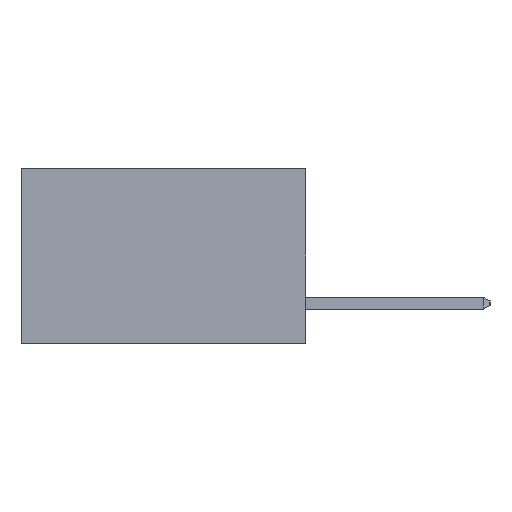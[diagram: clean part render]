
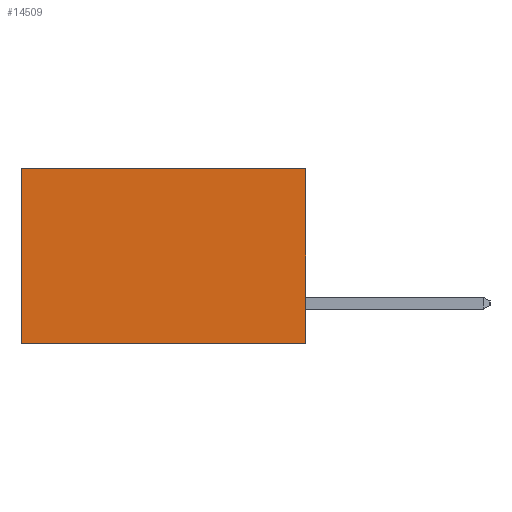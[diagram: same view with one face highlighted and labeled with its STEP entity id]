
A CAD part, left-side view. The second image highlights one B-rep face of the part: STEP entity #14509.
In plain terms, the highlighted planar face has unit normal (-1, 0, 0).
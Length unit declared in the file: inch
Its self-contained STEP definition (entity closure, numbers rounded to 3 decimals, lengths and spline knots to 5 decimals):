
#108 = ORIENTED_EDGE ( 'NONE', *, *, #2019, .T. ) ;
#853 = CARTESIAN_POINT ( 'NONE',  ( 0.298, 0.6, -0.37 ) ) ;
#903 = CARTESIAN_POINT ( 'NONE',  ( 0.298, 0., -0.37 ) ) ;
#1868 = CARTESIAN_POINT ( 'NONE',  ( 0.298, 0., 0. ) ) ;
#1919 = DIRECTION ( 'NONE',  ( 0., 0., -1. ) ) ;
#1975 = LINE ( 'NONE', #5694, #4301 ) ;
#2019 = EDGE_CURVE ( 'NONE', #9309, #12048, #1975, .T. ) ;
#2852 = VERTEX_POINT ( 'NONE', #903 ) ;
#3223 = DIRECTION ( 'NONE',  ( 0., 0., -1. ) ) ;
#3335 = CARTESIAN_POINT ( 'NONE',  ( 0.298, 0.6, 0. ) ) ;
#4014 = VECTOR ( 'NONE', #3223, 39.37008 ) ;
#4079 = EDGE_CURVE ( 'NONE', #2852, #15854, #13560, .T. ) ;
#4191 = ORIENTED_EDGE ( 'NONE', *, *, #8934, .F. ) ;
#4301 = VECTOR ( 'NONE', #5587, 39.37008 ) ;
#4930 = EDGE_LOOP ( 'NONE', ( #15391, #8726, #4191, #108 ) ) ;
#5587 = DIRECTION ( 'NONE',  ( 0., 1., 0. ) ) ;
#5694 = CARTESIAN_POINT ( 'NONE',  ( 0.298, 0., 0. ) ) ;
#6386 = CARTESIAN_POINT ( 'NONE',  ( 0.298, 0., 0. ) ) ;
#6669 = EDGE_CURVE ( 'NONE', #12048, #15854, #7245, .T. ) ;
#7245 = LINE ( 'NONE', #3335, #14487 ) ;
#7511 = LINE ( 'NONE', #1868, #4014 ) ;
#7709 = DIRECTION ( 'NONE',  ( 1., 0., 0. ) ) ;
#8726 = ORIENTED_EDGE ( 'NONE', *, *, #4079, .F. ) ;
#8934 = EDGE_CURVE ( 'NONE', #9309, #2852, #7511, .T. ) ;
#9309 = VERTEX_POINT ( 'NONE', #14478 ) ;
#9918 = FACE_OUTER_BOUND ( 'NONE', #4930, .T. ) ;
#10543 = VECTOR ( 'NONE', #13868, 39.37008 ) ;
#12048 = VERTEX_POINT ( 'NONE', #16599 ) ;
#12808 = AXIS2_PLACEMENT_3D ( 'NONE', #6386, #7709, #16581 ) ;
#13560 = LINE ( 'NONE', #13883, #10543 ) ;
#13868 = DIRECTION ( 'NONE',  ( 0., 1., 0. ) ) ;
#13883 = CARTESIAN_POINT ( 'NONE',  ( 0.298, 0., -0.37 ) ) ;
#14102 = PLANE ( 'NONE',  #12808 ) ;
#14478 = CARTESIAN_POINT ( 'NONE',  ( 0.298, 0., 0. ) ) ;
#14487 = VECTOR ( 'NONE', #1919, 39.37008 ) ;
#14509 = ADVANCED_FACE ( 'NONE', ( #9918 ), #14102, .F. ) ;
#15391 = ORIENTED_EDGE ( 'NONE', *, *, #6669, .T. ) ;
#15854 = VERTEX_POINT ( 'NONE', #853 ) ;
#16581 = DIRECTION ( 'NONE',  ( 0., 0., -1. ) ) ;
#16599 = CARTESIAN_POINT ( 'NONE',  ( 0.298, 0.6, 0. ) ) ;
